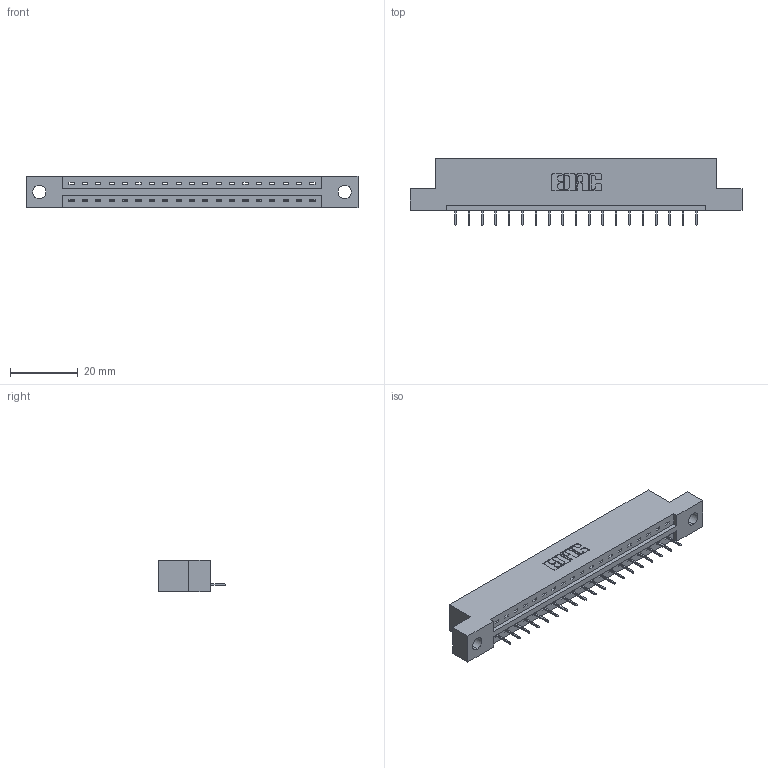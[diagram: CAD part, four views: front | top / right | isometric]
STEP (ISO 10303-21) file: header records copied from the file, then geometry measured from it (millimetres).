
FILE_DESCRIPTION (( 'STEP AP203' ), '1' );
FILE_NAME ('337-019-524-104.STEP', '2018-08-05T07:07:54', ( '' ), ( '' ), 'SwSTEP 2.0', 'SolidWorks 2016', '' );
FILE_SCHEMA (( 'CONFIG_CONTROL_DESIGN' ));
Length unit declared in the file: inch
Products named in the file (3): 337-019-524-104; 337 Part_Flush Mounting Lugs - 0.156 Dia-TH; 345-292-001_345-293-124
Assembly tree (20 placements, depth 2):
  337-019-524-104
    337 Part_Flush Mounting Lugs - 0.156 Dia-TH
    345-292-001_345-293-124  x19
Bounding box: 98.3 x 19.69 x 9.4 mm (x, y, z)
Volume: 9765.7 mm3; surface area: 9495.1 mm2
Topology: 20 solids, 20 shells, 1368 faces, 3959 edges, 2562 vertices
Faces by surface type: plane 1058, cylinder 310
Entity records: 17175 total; most frequent: CARTESIAN_POINT 2995, ORIENTED_EDGE 2950, DIRECTION 2569, EDGE_CURVE 1475, VECTOR 1351, LINE 1351, VERTEX_POINT 978, AXIS2_PLACEMENT_3D 609
